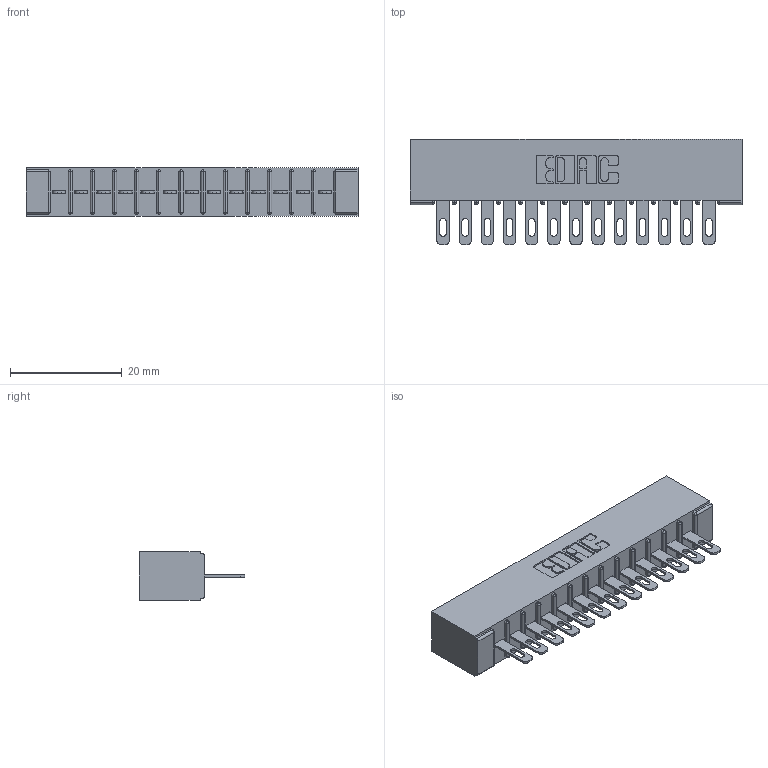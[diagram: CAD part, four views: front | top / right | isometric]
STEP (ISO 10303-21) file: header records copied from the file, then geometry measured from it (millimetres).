
FILE_DESCRIPTION (( 'STEP AP203' ), '1' );
FILE_NAME ('316-013-400-101.STEP', '2020-09-22T16:19:49', ( '' ), ( '' ), 'SwSTEP 2.0', 'SolidWorks 2020', '' );
FILE_SCHEMA (( 'CONFIG_CONTROL_DESIGN' ));
Length unit declared in the file: inch
Products named in the file (3): 316-013-400-101; 306-290-001_100; 306 Part_No Mounting
Assembly tree (14 placements, depth 2):
  316-013-400-101
    306 Part_No Mounting
    306-290-001_100  x13
Bounding box: 59.39 x 18.87 x 8.71 mm (x, y, z)
Volume: 4344.2 mm3; surface area: 6595.5 mm2
Topology: 14 solids, 14 shells, 1096 faces, 3087 edges, 1986 vertices
Faces by surface type: plane 714, cylinder 330, sphere 52
Entity records: 15766 total; most frequent: CARTESIAN_POINT 2642, ORIENTED_EDGE 2614, DIRECTION 2609, EDGE_CURVE 1307, VECTOR 1007, LINE 1007, VERTEX_POINT 834, AXIS2_PLACEMENT_3D 801
